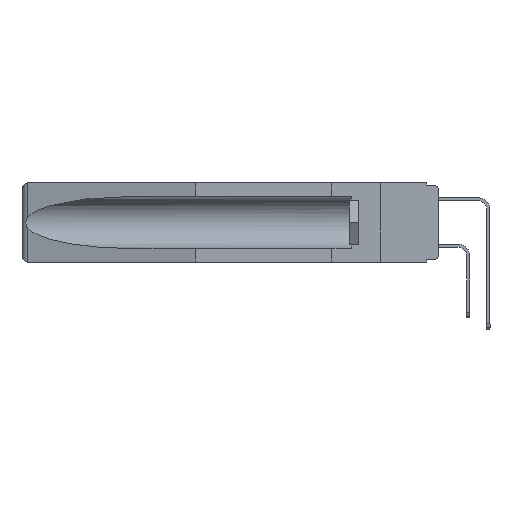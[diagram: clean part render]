
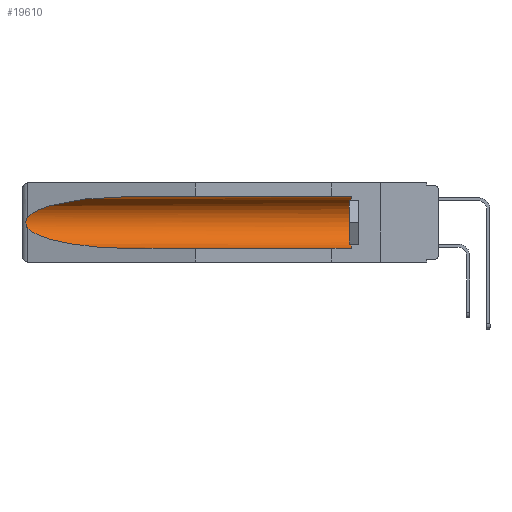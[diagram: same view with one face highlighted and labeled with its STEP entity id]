
A CAD part, left-side view. The second image highlights one B-rep face of the part: STEP entity #19610.
In plain terms, the highlighted cylindrical face has radius 2.857 mm (diameter 5.715 mm), a partial arc.
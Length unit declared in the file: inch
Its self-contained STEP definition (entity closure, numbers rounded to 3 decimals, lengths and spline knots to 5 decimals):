
#249 = EDGE_LOOP ( 'NONE', ( #11976, #16718, #21274, #19724, #18374, #20547 ) ) ;
#587 = LINE ( 'NONE', #5434, #19687 ) ;
#1505 = CARTESIAN_POINT ( 'NONE',  ( 0.2675, 1.53308, -0.17534 ) ) ;
#1932 = CARTESIAN_POINT ( 'NONE',  ( 0.155, 0.126, -0.1715 ) ) ;
#2036 = DIRECTION ( 'NONE',  ( 0., 0., 1. ) ) ;
#2088 = EDGE_CURVE ( 'NONE', #14826, #6592, #3496, .T. ) ;
#2309 = DIRECTION ( 'NONE',  ( 0., 1., 0. ) ) ;
#2978 = DIRECTION ( 'NONE',  ( 0., 0., 1. ) ) ;
#3151 = VERTEX_POINT ( 'NONE', #5740 ) ;
#3182 = CARTESIAN_POINT ( 'NONE',  ( 0.26537, 1.52718, -0.14972 ) ) ;
#3496 = CIRCLE ( 'NONE', #3515, 0.1125 ) ;
#3515 = AXIS2_PLACEMENT_3D ( 'NONE', #1932, #16804, #2036 ) ;
#4045 = CARTESIAN_POINT ( 'NONE',  ( 0.21114, 1.30732, -0.284 ) ) ;
#4168 = VERTEX_POINT ( 'NONE', #3182 ) ;
#4415 = CARTESIAN_POINT ( 'NONE',  ( 0.26537, 1.52718, -0.14972 ) ) ;
#4604 = CYLINDRICAL_SURFACE ( 'NONE', #7901, 0.1125 ) ;
#5413 = EDGE_CURVE ( 'NONE', #4168, #15462, #16121, .T. ) ;
#5434 = CARTESIAN_POINT ( 'NONE',  ( 0.155, -0.30754, -0.284 ) ) ;
#5740 = CARTESIAN_POINT ( 'NONE',  ( 0.155, 1.07973, -0.284 ) ) ;
#5790 = CARTESIAN_POINT ( 'NONE',  ( 0.21114, 1.30732, -0.059 ) ) ;
#5807 = CARTESIAN_POINT ( 'NONE',  ( 0.155, 0.126, -0.284 ) ) ;
#5961 = CARTESIAN_POINT ( 'NONE',  ( 0.155, 0.126, -0.059 ) ) ;
#6079 = EDGE_CURVE ( 'NONE', #15773, #4168, #19287, .T. ) ;
#6120 = CARTESIAN_POINT ( 'NONE',  ( 0.2675, 1.53308, -0.16763 ) ) ;
#6347 = CARTESIAN_POINT ( 'NONE',  ( 0.26655, 1.53094, -0.18657 ) ) ;
#6592 = VERTEX_POINT ( 'NONE', #5961 ) ;
#7201 = CARTESIAN_POINT ( 'NONE',  ( 0.26537, 1.52718, -0.14972 ) ) ;
#7901 = AXIS2_PLACEMENT_3D ( 'NONE', #12696, #20704, #2978 ) ;
#8336 = CARTESIAN_POINT ( 'NONE',  ( 0.26537, 1.52718, -0.19328 ) ) ;
#9330 = DIRECTION ( 'NONE',  ( 0., 1., 0. ) ) ;
#9648 =( BOUNDED_CURVE ( )  B_SPLINE_CURVE ( 3, ( #15270, #15589, #4045, #16890 ),
 .UNSPECIFIED., .F., .F. ) 
 B_SPLINE_CURVE_WITH_KNOTS ( ( 4, 4 ),
 ( 0.1948, 1.5708 ),
 .UNSPECIFIED. ) 
 CURVE ( )  GEOMETRIC_REPRESENTATION_ITEM ( )  RATIONAL_B_SPLINE_CURVE ( ( 1., 0.848, 0.848, 1. ) ) 
 REPRESENTATION_ITEM ( '' )  );
#10744 = FACE_OUTER_BOUND ( 'NONE', #249, .T. ) ;
#11131 = CARTESIAN_POINT ( 'NONE',  ( 0.155, 1.07973, -0.059 ) ) ;
#11299 = CARTESIAN_POINT ( 'NONE',  ( 0.26654, 1.53092, -0.15636 ) ) ;
#11976 = ORIENTED_EDGE ( 'NONE', *, *, #6079, .T. ) ;
#12696 = CARTESIAN_POINT ( 'NONE',  ( 0.155, -0.30754, -0.1715 ) ) ;
#14074 = CARTESIAN_POINT ( 'NONE',  ( 0.155, -0.30754, -0.059 ) ) ;
#14443 = CARTESIAN_POINT ( 'NONE',  ( 0.2673, 1.53269, -0.17917 ) ) ;
#14660 = CARTESIAN_POINT ( 'NONE',  ( 0.26537, 1.52718, -0.19328 ) ) ;
#14826 = VERTEX_POINT ( 'NONE', #5807 ) ;
#15270 = CARTESIAN_POINT ( 'NONE',  ( 0.26537, 1.52718, -0.19328 ) ) ;
#15462 = VERTEX_POINT ( 'NONE', #8336 ) ;
#15589 = CARTESIAN_POINT ( 'NONE',  ( 0.25451, 1.48313, -0.24835 ) ) ;
#15773 = VERTEX_POINT ( 'NONE', #11131 ) ;
#15848 = CARTESIAN_POINT ( 'NONE',  ( 0.26597, 1.5296, -0.19026 ) ) ;
#16060 = CARTESIAN_POINT ( 'NONE',  ( 0.26597, 1.52961, -0.15275 ) ) ;
#16121 = B_SPLINE_CURVE_WITH_KNOTS ( 'NONE', 3,
 ( #4415, #16060, #11299, #17895, #6120, #1505, #14443, #6347, #15848, #14660 ),
 .UNSPECIFIED., .F., .F.,
 ( 4, 2, 2, 2, 4 ),
 ( 0., 0.00029, 0.00058, 0.00087, 0.00117 ),
 .UNSPECIFIED. ) ;
#16718 = ORIENTED_EDGE ( 'NONE', *, *, #5413, .T. ) ;
#16804 = DIRECTION ( 'NONE',  ( 0., -1., 0. ) ) ;
#16890 = CARTESIAN_POINT ( 'NONE',  ( 0.155, 1.07973, -0.284 ) ) ;
#16934 = EDGE_CURVE ( 'NONE', #15462, #3151, #9648, .T. ) ;
#17055 = EDGE_CURVE ( 'NONE', #6592, #15773, #19061, .T. ) ;
#17895 = CARTESIAN_POINT ( 'NONE',  ( 0.2673, 1.5327, -0.16383 ) ) ;
#18374 = ORIENTED_EDGE ( 'NONE', *, *, #2088, .T. ) ;
#18983 = CARTESIAN_POINT ( 'NONE',  ( 0.155, 1.07973, -0.059 ) ) ;
#19061 = LINE ( 'NONE', #14074, #19279 ) ;
#19279 = VECTOR ( 'NONE', #9330, 39.37008 ) ;
#19287 =( BOUNDED_CURVE ( )  B_SPLINE_CURVE ( 3, ( #18983, #5790, #20401, #7201 ),
 .UNSPECIFIED., .F., .F. ) 
 B_SPLINE_CURVE_WITH_KNOTS ( ( 4, 4 ),
 ( 4.71239, 6.08839 ),
 .UNSPECIFIED. ) 
 CURVE ( )  GEOMETRIC_REPRESENTATION_ITEM ( )  RATIONAL_B_SPLINE_CURVE ( ( 1., 0.848, 0.848, 1. ) ) 
 REPRESENTATION_ITEM ( '' )  );
#19610 = ADVANCED_FACE ( 'NONE', ( #10744 ), #4604, .F. ) ;
#19687 = VECTOR ( 'NONE', #2309, 39.37008 ) ;
#19724 = ORIENTED_EDGE ( 'NONE', *, *, #21264, .F. ) ;
#20401 = CARTESIAN_POINT ( 'NONE',  ( 0.25451, 1.48313, -0.09465 ) ) ;
#20547 = ORIENTED_EDGE ( 'NONE', *, *, #17055, .T. ) ;
#20704 = DIRECTION ( 'NONE',  ( 0., 1., 0. ) ) ;
#21264 = EDGE_CURVE ( 'NONE', #14826, #3151, #587, .T. ) ;
#21274 = ORIENTED_EDGE ( 'NONE', *, *, #16934, .T. ) ;
